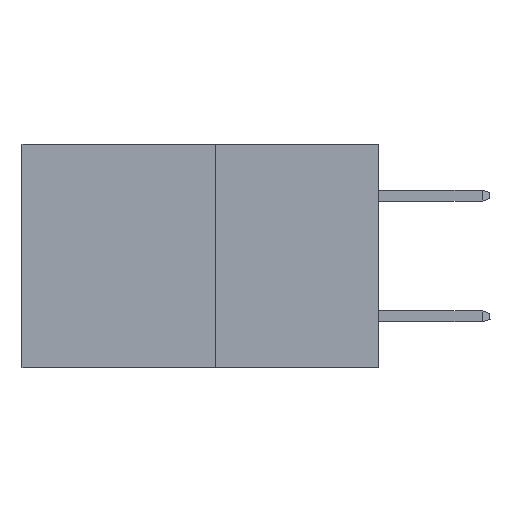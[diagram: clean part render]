
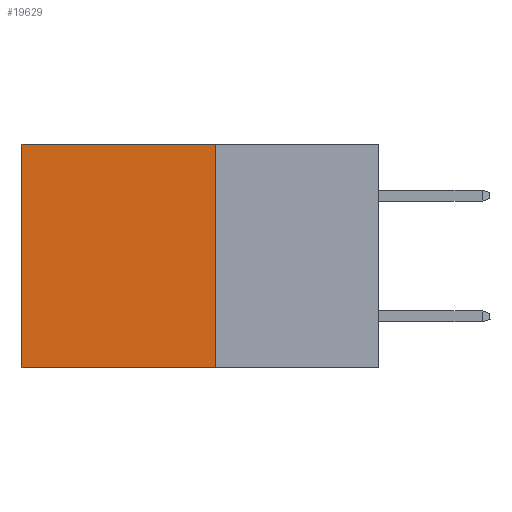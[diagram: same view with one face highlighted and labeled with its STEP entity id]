
A CAD part, left-side view. The second image highlights one B-rep face of the part: STEP entity #19629.
In plain terms, the highlighted planar face has unit normal (-1, 0, 0).
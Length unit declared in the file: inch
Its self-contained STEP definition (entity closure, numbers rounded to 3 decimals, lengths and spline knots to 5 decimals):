
#811 = CARTESIAN_POINT ( 'NONE',  ( 0.277, 0.59, 0. ) ) ;
#1078 = PLANE ( 'NONE',  #2334 ) ;
#1527 = EDGE_CURVE ( 'NONE', #17408, #6637, #23573, .T. ) ;
#2334 = AXIS2_PLACEMENT_3D ( 'NONE', #3077, #4982, #18297 ) ;
#3077 = CARTESIAN_POINT ( 'NONE',  ( 0.277, 0.27, -0.37 ) ) ;
#4982 = DIRECTION ( 'NONE',  ( 1., 0., 0. ) ) ;
#5556 = EDGE_CURVE ( 'NONE', #17408, #21453, #18693, .T. ) ;
#5701 = EDGE_CURVE ( 'NONE', #6637, #10920, #15971, .T. ) ;
#5748 = ORIENTED_EDGE ( 'NONE', *, *, #5556, .F. ) ;
#5765 = CARTESIAN_POINT ( 'NONE',  ( 0.277, 0.59, -0.37 ) ) ;
#5868 = EDGE_LOOP ( 'NONE', ( #8332, #23984, #5748, #18520 ) ) ;
#6062 = CARTESIAN_POINT ( 'NONE',  ( 0.277, 0.27, 0. ) ) ;
#6637 = VERTEX_POINT ( 'NONE', #811 ) ;
#8224 = LINE ( 'NONE', #13532, #22225 ) ;
#8332 = ORIENTED_EDGE ( 'NONE', *, *, #5701, .T. ) ;
#10494 = CARTESIAN_POINT ( 'NONE',  ( 0.277, 0.59, -0.37 ) ) ;
#10920 = VERTEX_POINT ( 'NONE', #10494 ) ;
#10926 = VECTOR ( 'NONE', #22878, 39.37008 ) ;
#13008 = DIRECTION ( 'NONE',  ( 0., 0., -1. ) ) ;
#13532 = CARTESIAN_POINT ( 'NONE',  ( 0.277, 0.27, -0.37 ) ) ;
#13600 = VECTOR ( 'NONE', #13008, 39.37008 ) ;
#14907 = CARTESIAN_POINT ( 'NONE',  ( 0.277, 0.27, -0.37 ) ) ;
#15459 = DIRECTION ( 'NONE',  ( 0., 1., 0. ) ) ;
#15691 = CARTESIAN_POINT ( 'NONE',  ( 0.277, 0.27, 0. ) ) ;
#15971 = LINE ( 'NONE', #5765, #10926 ) ;
#16447 = FACE_OUTER_BOUND ( 'NONE', #5868, .T. ) ;
#17313 = DIRECTION ( 'NONE',  ( 0., 1., 0. ) ) ;
#17408 = VERTEX_POINT ( 'NONE', #6062 ) ;
#17933 = VECTOR ( 'NONE', #17313, 39.37008 ) ;
#18297 = DIRECTION ( 'NONE',  ( 0., 0., -1. ) ) ;
#18520 = ORIENTED_EDGE ( 'NONE', *, *, #1527, .T. ) ;
#18693 = LINE ( 'NONE', #14907, #13600 ) ;
#19629 = ADVANCED_FACE ( 'NONE', ( #16447 ), #1078, .F. ) ;
#21453 = VERTEX_POINT ( 'NONE', #23197 ) ;
#22070 = EDGE_CURVE ( 'NONE', #21453, #10920, #8224, .T. ) ;
#22225 = VECTOR ( 'NONE', #15459, 39.37008 ) ;
#22878 = DIRECTION ( 'NONE',  ( 0., 0., -1. ) ) ;
#23197 = CARTESIAN_POINT ( 'NONE',  ( 0.277, 0.27, -0.37 ) ) ;
#23573 = LINE ( 'NONE', #15691, #17933 ) ;
#23984 = ORIENTED_EDGE ( 'NONE', *, *, #22070, .F. ) ;
